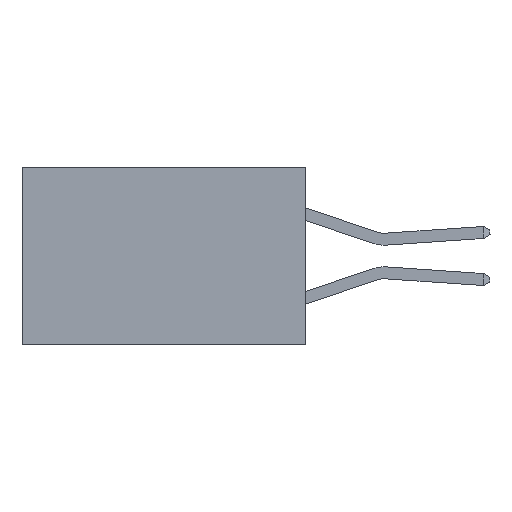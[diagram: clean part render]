
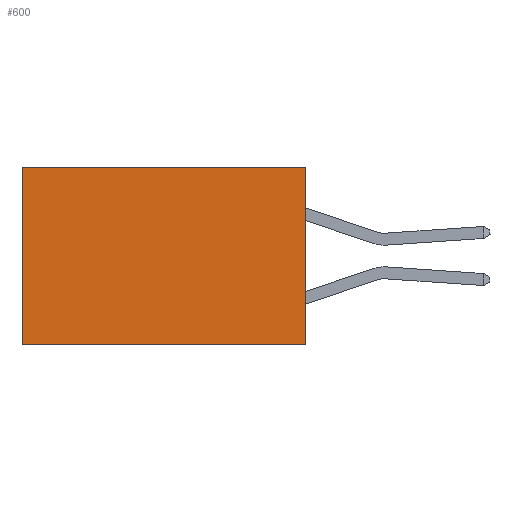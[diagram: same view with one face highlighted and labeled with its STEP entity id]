
A CAD part, left-side view. The second image highlights one B-rep face of the part: STEP entity #600.
In plain terms, the highlighted planar face has unit normal (-1, 0, 0).
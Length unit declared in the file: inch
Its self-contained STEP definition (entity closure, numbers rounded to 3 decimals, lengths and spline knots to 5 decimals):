
#600 = ADVANCED_FACE ( 'NONE', ( #4717 ), #6477, .F. ) ;
#617 = DIRECTION ( 'NONE',  ( 1., 0., 0. ) ) ;
#770 = CARTESIAN_POINT ( 'NONE',  ( 0.277, 0., 0. ) ) ;
#902 = CARTESIAN_POINT ( 'NONE',  ( 0.277, 0., -0.37 ) ) ;
#1149 = ORIENTED_EDGE ( 'NONE', *, *, #3272, .T. ) ;
#1303 = LINE ( 'NONE', #770, #3242 ) ;
#1314 = ORIENTED_EDGE ( 'NONE', *, *, #5235, .F. ) ;
#1342 = ORIENTED_EDGE ( 'NONE', *, *, #3614, .F. ) ;
#1397 = ORIENTED_EDGE ( 'NONE', *, *, #4502, .T. ) ;
#1812 = DIRECTION ( 'NONE',  ( 0., 0., -1. ) ) ;
#1922 = CARTESIAN_POINT ( 'NONE',  ( 0.277, 0.59, 0. ) ) ;
#2141 = CARTESIAN_POINT ( 'NONE',  ( 0.277, 0., -0.37 ) ) ;
#2277 = VECTOR ( 'NONE', #9498, 39.37008 ) ;
#2500 = DIRECTION ( 'NONE',  ( 0., 0., -1. ) ) ;
#2524 = LINE ( 'NONE', #4738, #6515 ) ;
#3242 = VECTOR ( 'NONE', #4019, 39.37008 ) ;
#3265 = CARTESIAN_POINT ( 'NONE',  ( 0.277, 0., -0.37 ) ) ;
#3272 = EDGE_CURVE ( 'NONE', #4863, #4029, #2524, .T. ) ;
#3614 = EDGE_CURVE ( 'NONE', #9591, #5026, #6279, .T. ) ;
#3678 = VECTOR ( 'NONE', #8167, 39.37008 ) ;
#4019 = DIRECTION ( 'NONE',  ( 0., 1., 0. ) ) ;
#4029 = VERTEX_POINT ( 'NONE', #4439 ) ;
#4439 = CARTESIAN_POINT ( 'NONE',  ( 0.277, 0.59, -0.37 ) ) ;
#4502 = EDGE_CURVE ( 'NONE', #9591, #4863, #1303, .T. ) ;
#4531 = CARTESIAN_POINT ( 'NONE',  ( 0.277, 0., 0. ) ) ;
#4717 = FACE_OUTER_BOUND ( 'NONE', #7205, .T. ) ;
#4738 = CARTESIAN_POINT ( 'NONE',  ( 0.277, 0.59, -0.37 ) ) ;
#4863 = VERTEX_POINT ( 'NONE', #1922 ) ;
#5026 = VERTEX_POINT ( 'NONE', #3265 ) ;
#5235 = EDGE_CURVE ( 'NONE', #5026, #4029, #7531, .T. ) ;
#5381 = AXIS2_PLACEMENT_3D ( 'NONE', #902, #617, #2500 ) ;
#6279 = LINE ( 'NONE', #2141, #2277 ) ;
#6477 = PLANE ( 'NONE',  #5381 ) ;
#6515 = VECTOR ( 'NONE', #1812, 39.37008 ) ;
#7205 = EDGE_LOOP ( 'NONE', ( #1149, #1314, #1342, #1397 ) ) ;
#7531 = LINE ( 'NONE', #8029, #3678 ) ;
#8029 = CARTESIAN_POINT ( 'NONE',  ( 0.277, 0., -0.37 ) ) ;
#8167 = DIRECTION ( 'NONE',  ( 0., 1., 0. ) ) ;
#9498 = DIRECTION ( 'NONE',  ( 0., 0., -1. ) ) ;
#9591 = VERTEX_POINT ( 'NONE', #4531 ) ;
